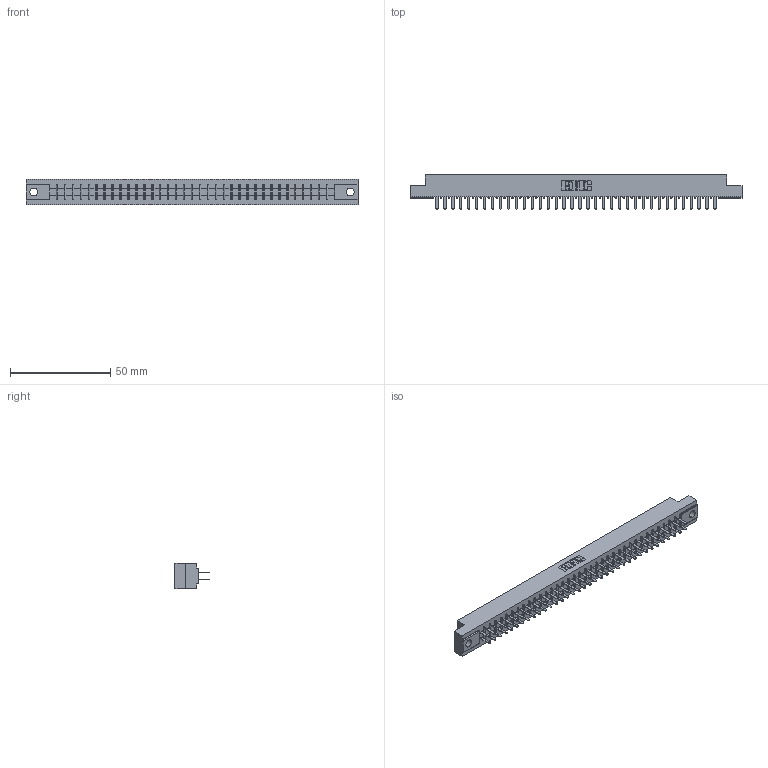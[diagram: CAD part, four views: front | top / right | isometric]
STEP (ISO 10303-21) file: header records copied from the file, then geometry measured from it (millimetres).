
FILE_DESCRIPTION (( 'STEP AP203' ), '1' );
FILE_NAME ('315-072-520-204.STEP', '2019-09-10T21:44:15', ( '' ), ( '' ), 'SwSTEP 2.0', 'SolidWorks 2016', '' );
FILE_SCHEMA (( 'CONFIG_CONTROL_DESIGN' ));
Length unit declared in the file: inch
Products named in the file (3): 315-072-520-204; 305-290-001_520; 305 Part_.156 Dia
Assembly tree (73 placements, depth 2):
  315-072-520-204
    305 Part_.156 Dia
    305-290-001_520  x72
Bounding box: 165.66 x 17.09 x 12.7 mm (x, y, z)
Volume: 17136.7 mm3; surface area: 21552.1 mm2
Topology: 73 solids, 73 shells, 3442 faces, 9820 edges, 6352 vertices
Faces by surface type: plane 2026, cylinder 1272, sphere 144
Entity records: 40007 total; most frequent: CARTESIAN_POINT 6624, ORIENTED_EDGE 6572, DIRECTION 6404, EDGE_CURVE 3286, LINE 2660, VECTOR 2660, VERTEX_POINT 2092, AXIS2_PLACEMENT_3D 1872
